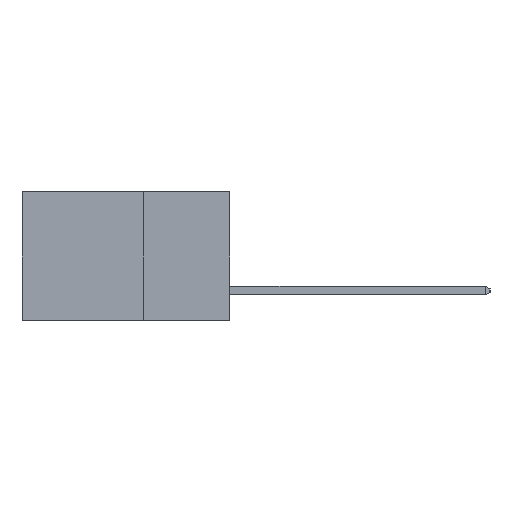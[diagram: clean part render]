
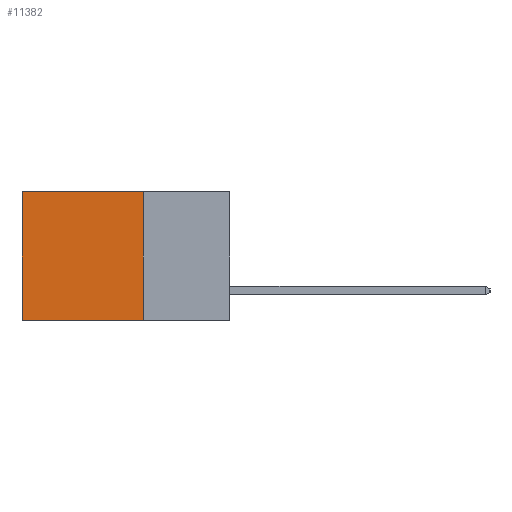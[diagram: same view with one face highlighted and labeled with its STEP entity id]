
A CAD part, left-side view. The second image highlights one B-rep face of the part: STEP entity #11382.
In plain terms, the highlighted planar face has unit normal (-1, 0, 0).
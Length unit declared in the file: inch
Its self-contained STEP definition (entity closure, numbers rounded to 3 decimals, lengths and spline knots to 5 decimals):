
#155 = CARTESIAN_POINT ( 'NONE',  ( 0.2615, 0.25, -0.37 ) ) ;
#202 = ORIENTED_EDGE ( 'NONE', *, *, #21645, .T. ) ;
#307 = VECTOR ( 'NONE', #5826, 39.37008 ) ;
#1219 = DIRECTION ( 'NONE',  ( 0., 1., 0. ) ) ;
#1418 = CARTESIAN_POINT ( 'NONE',  ( 0.2615, 0.25, -0.37 ) ) ;
#1774 = CARTESIAN_POINT ( 'NONE',  ( 0.2615, 0.25, 0. ) ) ;
#1990 = EDGE_LOOP ( 'NONE', ( #11094, #19008, #15245, #202 ) ) ;
#3389 = DIRECTION ( 'NONE',  ( 1., 0., 0. ) ) ;
#3677 = EDGE_CURVE ( 'NONE', #21284, #20389, #15805, .T. ) ;
#4693 = DIRECTION ( 'NONE',  ( 0., 0., -1. ) ) ;
#4914 = VECTOR ( 'NONE', #5239, 39.37008 ) ;
#5101 = PLANE ( 'NONE',  #19473 ) ;
#5239 = DIRECTION ( 'NONE',  ( 0., 1., 0. ) ) ;
#5826 = DIRECTION ( 'NONE',  ( 0., 0., -1. ) ) ;
#5853 = CARTESIAN_POINT ( 'NONE',  ( 0.2615, 0.6, -0.37 ) ) ;
#8416 = DIRECTION ( 'NONE',  ( 0., 0., -1. ) ) ;
#8454 = CARTESIAN_POINT ( 'NONE',  ( 0.2615, 0.25, -0.37 ) ) ;
#11094 = ORIENTED_EDGE ( 'NONE', *, *, #3677, .T. ) ;
#11316 = VERTEX_POINT ( 'NONE', #22822 ) ;
#11382 = ADVANCED_FACE ( 'NONE', ( #22685 ), #5101, .F. ) ;
#11503 = LINE ( 'NONE', #16639, #15990 ) ;
#15245 = ORIENTED_EDGE ( 'NONE', *, *, #16576, .F. ) ;
#15265 = EDGE_CURVE ( 'NONE', #11316, #20389, #20152, .T. ) ;
#15642 = CARTESIAN_POINT ( 'NONE',  ( 0.2615, 0.6, 0. ) ) ;
#15805 = LINE ( 'NONE', #5853, #307 ) ;
#15990 = VECTOR ( 'NONE', #1219, 39.37008 ) ;
#16576 = EDGE_CURVE ( 'NONE', #22419, #11316, #18382, .T. ) ;
#16639 = CARTESIAN_POINT ( 'NONE',  ( 0.2615, 0.25, 0. ) ) ;
#17620 = CARTESIAN_POINT ( 'NONE',  ( 0.2615, 0.6, -0.37 ) ) ;
#18382 = LINE ( 'NONE', #8454, #24238 ) ;
#19008 = ORIENTED_EDGE ( 'NONE', *, *, #15265, .F. ) ;
#19473 = AXIS2_PLACEMENT_3D ( 'NONE', #1418, #3389, #4693 ) ;
#20152 = LINE ( 'NONE', #155, #4914 ) ;
#20389 = VERTEX_POINT ( 'NONE', #17620 ) ;
#21284 = VERTEX_POINT ( 'NONE', #15642 ) ;
#21645 = EDGE_CURVE ( 'NONE', #22419, #21284, #11503, .T. ) ;
#22419 = VERTEX_POINT ( 'NONE', #1774 ) ;
#22685 = FACE_OUTER_BOUND ( 'NONE', #1990, .T. ) ;
#22822 = CARTESIAN_POINT ( 'NONE',  ( 0.2615, 0.25, -0.37 ) ) ;
#24238 = VECTOR ( 'NONE', #8416, 39.37008 ) ;
